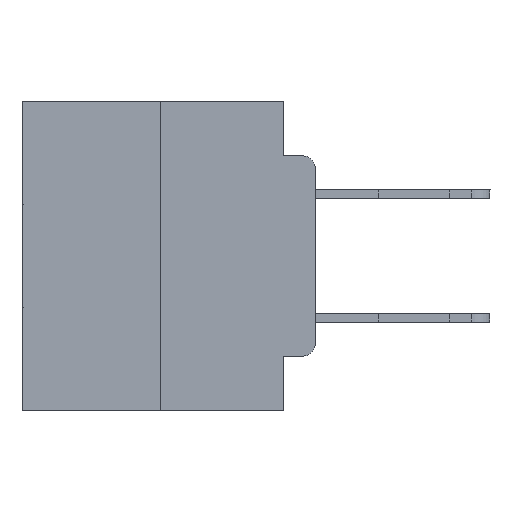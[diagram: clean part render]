
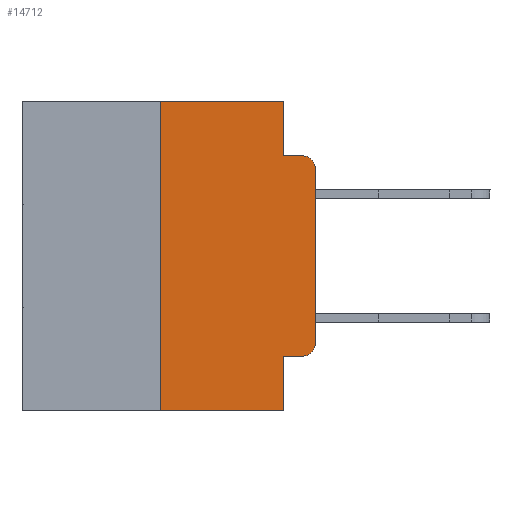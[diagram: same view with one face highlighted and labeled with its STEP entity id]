
A CAD part, left-side view. The second image highlights one B-rep face of the part: STEP entity #14712.
In plain terms, the highlighted planar face has unit normal (-1, 0, 0).
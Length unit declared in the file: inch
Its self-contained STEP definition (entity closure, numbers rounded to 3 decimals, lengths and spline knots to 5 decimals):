
#131 = CARTESIAN_POINT ( 'NONE',  ( 0., 0.02, -0.4115 ) ) ;
#291 = CARTESIAN_POINT ( 'NONE',  ( 0., 0.473, 0. ) ) ;
#355 = CARTESIAN_POINT ( 'NONE',  ( 0., 0.051, -0.0885 ) ) ;
#356 = VECTOR ( 'NONE', #28838, 39.37008 ) ;
#1046 = LINE ( 'NONE', #3327, #4243 ) ;
#1281 = CARTESIAN_POINT ( 'NONE',  ( 0., 0.473, 0. ) ) ;
#1466 = DIRECTION ( 'NONE',  ( 0., 0., -1. ) ) ;
#1649 = CARTESIAN_POINT ( 'NONE',  ( 0., 0.02, -0.0885 ) ) ;
#1907 = ORIENTED_EDGE ( 'NONE', *, *, #23450, .F. ) ;
#1932 = ORIENTED_EDGE ( 'NONE', *, *, #23886, .F. ) ;
#2139 = EDGE_CURVE ( 'NONE', #19754, #22920, #22106, .T. ) ;
#2626 = VERTEX_POINT ( 'NONE', #25059 ) ;
#2666 = FACE_OUTER_BOUND ( 'NONE', #6830, .T. ) ;
#3076 = DIRECTION ( 'NONE',  ( 0., 0., -1. ) ) ;
#3327 = CARTESIAN_POINT ( 'NONE',  ( 0., 0.051, 0. ) ) ;
#4243 = VECTOR ( 'NONE', #21700, 39.37008 ) ;
#4578 = EDGE_CURVE ( 'NONE', #19847, #6266, #21997, .T. ) ;
#4613 = VERTEX_POINT ( 'NONE', #28616 ) ;
#4696 = ORIENTED_EDGE ( 'NONE', *, *, #9099, .T. ) ;
#5130 = AXIS2_PLACEMENT_3D ( 'NONE', #16381, #12075, #3076 ) ;
#6266 = VERTEX_POINT ( 'NONE', #1649 ) ;
#6611 = CARTESIAN_POINT ( 'NONE',  ( 0., 0.473, -0.5 ) ) ;
#6830 = EDGE_LOOP ( 'NONE', ( #24484, #16976, #23348, #7149, #20069, #1907, #4696, #1932, #20699, #22631 ) ) ;
#6995 = LINE ( 'NONE', #25992, #10140 ) ;
#7149 = ORIENTED_EDGE ( 'NONE', *, *, #9738, .F. ) ;
#7363 = LINE ( 'NONE', #11309, #356 ) ;
#7456 = CARTESIAN_POINT ( 'NONE',  ( 0., 0.051, -0.0885 ) ) ;
#7918 = CARTESIAN_POINT ( 'NONE',  ( 0., 0.051, -0.4115 ) ) ;
#8539 = CARTESIAN_POINT ( 'NONE',  ( 0., 0.02, -0.1085 ) ) ;
#8569 = CIRCLE ( 'NONE', #5130, 0.02 ) ;
#8651 = DIRECTION ( 'NONE',  ( 0., -1., 0. ) ) ;
#8864 = VERTEX_POINT ( 'NONE', #25711 ) ;
#9099 = EDGE_CURVE ( 'NONE', #18301, #2626, #9167, .T. ) ;
#9167 = LINE ( 'NONE', #6611, #12659 ) ;
#9738 = EDGE_CURVE ( 'NONE', #22920, #15021, #1046, .T. ) ;
#10140 = VECTOR ( 'NONE', #1466, 39.37008 ) ;
#10187 = DIRECTION ( 'NONE',  ( 0., -1., 0. ) ) ;
#10406 = PLANE ( 'NONE',  #15418 ) ;
#11309 = CARTESIAN_POINT ( 'NONE',  ( 0., 0.25, 0. ) ) ;
#11358 = VECTOR ( 'NONE', #19634, 39.37008 ) ;
#11532 = AXIS2_PLACEMENT_3D ( 'NONE', #8539, #13029, #24045 ) ;
#12075 = DIRECTION ( 'NONE',  ( -1., 0., 0. ) ) ;
#12659 = VECTOR ( 'NONE', #8651, 39.37008 ) ;
#13029 = DIRECTION ( 'NONE',  ( -1., 0., 0. ) ) ;
#13518 = LINE ( 'NONE', #7918, #14943 ) ;
#13853 = DIRECTION ( 'NONE',  ( 0., -1., 0. ) ) ;
#14658 = VECTOR ( 'NONE', #13853, 39.37008 ) ;
#14712 = ADVANCED_FACE ( 'NONE', ( #2666 ), #10406, .F. ) ;
#14943 = VECTOR ( 'NONE', #10187, 39.37008 ) ;
#15021 = VERTEX_POINT ( 'NONE', #7456 ) ;
#15157 = EDGE_CURVE ( 'NONE', #8864, #25344, #13518, .T. ) ;
#15418 = AXIS2_PLACEMENT_3D ( 'NONE', #1281, #16967, #23577 ) ;
#16279 = EDGE_CURVE ( 'NONE', #25344, #4613, #8569, .T. ) ;
#16381 = CARTESIAN_POINT ( 'NONE',  ( 0., 0.02, -0.3915 ) ) ;
#16967 = DIRECTION ( 'NONE',  ( 1., 0., 0. ) ) ;
#16976 = ORIENTED_EDGE ( 'NONE', *, *, #4578, .T. ) ;
#18092 = DIRECTION ( 'NONE',  ( 0., -1., 0. ) ) ;
#18301 = VERTEX_POINT ( 'NONE', #20148 ) ;
#19634 = DIRECTION ( 'NONE',  ( 0., 0., 1. ) ) ;
#19754 = VERTEX_POINT ( 'NONE', #22235 ) ;
#19844 = CARTESIAN_POINT ( 'NONE',  ( 0., 0.051, 0. ) ) ;
#19847 = VERTEX_POINT ( 'NONE', #22607 ) ;
#20069 = ORIENTED_EDGE ( 'NONE', *, *, #2139, .F. ) ;
#20148 = CARTESIAN_POINT ( 'NONE',  ( 0., 0.25, -0.5 ) ) ;
#20699 = ORIENTED_EDGE ( 'NONE', *, *, #15157, .T. ) ;
#21700 = DIRECTION ( 'NONE',  ( 0., 0., -1. ) ) ;
#21997 = CIRCLE ( 'NONE', #11532, 0.02 ) ;
#22106 = LINE ( 'NONE', #291, #27305 ) ;
#22235 = CARTESIAN_POINT ( 'NONE',  ( 0., 0.25, 0. ) ) ;
#22607 = CARTESIAN_POINT ( 'NONE',  ( 0., 0., -0.1085 ) ) ;
#22631 = ORIENTED_EDGE ( 'NONE', *, *, #16279, .T. ) ;
#22920 = VERTEX_POINT ( 'NONE', #19844 ) ;
#23305 = CARTESIAN_POINT ( 'NONE',  ( 0., 0., 0. ) ) ;
#23348 = ORIENTED_EDGE ( 'NONE', *, *, #24737, .F. ) ;
#23450 = EDGE_CURVE ( 'NONE', #18301, #19754, #7363, .T. ) ;
#23577 = DIRECTION ( 'NONE',  ( 0., 0., -1. ) ) ;
#23886 = EDGE_CURVE ( 'NONE', #8864, #2626, #6995, .T. ) ;
#24045 = DIRECTION ( 'NONE',  ( 0., 0., -1. ) ) ;
#24484 = ORIENTED_EDGE ( 'NONE', *, *, #27749, .T. ) ;
#24737 = EDGE_CURVE ( 'NONE', #15021, #6266, #26495, .T. ) ;
#25059 = CARTESIAN_POINT ( 'NONE',  ( 0., 0.051, -0.5 ) ) ;
#25344 = VERTEX_POINT ( 'NONE', #131 ) ;
#25711 = CARTESIAN_POINT ( 'NONE',  ( 0., 0.051, -0.4115 ) ) ;
#25992 = CARTESIAN_POINT ( 'NONE',  ( 0., 0.051, 0. ) ) ;
#26495 = LINE ( 'NONE', #355, #14658 ) ;
#27305 = VECTOR ( 'NONE', #18092, 39.37008 ) ;
#27726 = LINE ( 'NONE', #23305, #11358 ) ;
#27749 = EDGE_CURVE ( 'NONE', #4613, #19847, #27726, .T. ) ;
#28616 = CARTESIAN_POINT ( 'NONE',  ( 0., 0., -0.3915 ) ) ;
#28838 = DIRECTION ( 'NONE',  ( 0., 0., 1. ) ) ;
